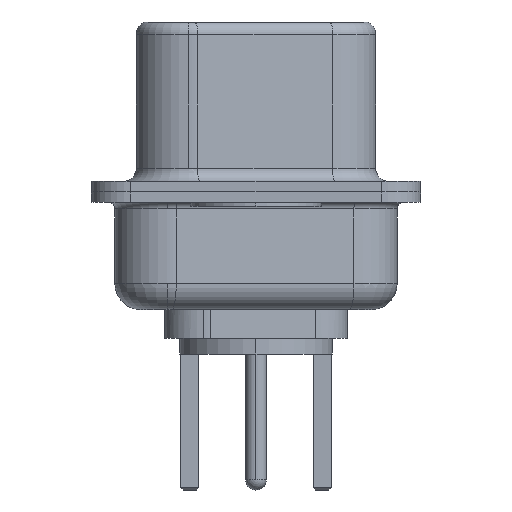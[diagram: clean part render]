
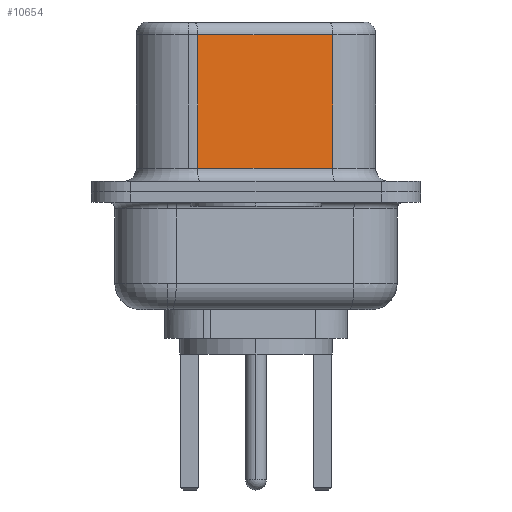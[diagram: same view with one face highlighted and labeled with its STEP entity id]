
A CAD part, left-side view. The second image highlights one B-rep face of the part: STEP entity #10654.
In plain terms, the highlighted planar face has unit normal (-0.985, -0.174, 0).
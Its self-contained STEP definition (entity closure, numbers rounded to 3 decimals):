
#803 = EDGE_LOOP ( 'NONE', ( #13712, #4889, #5428, #10880 ) ) ;
#1009 = VECTOR ( 'NONE', #5674, 1000. ) ;
#1105 = VECTOR ( 'NONE', #13350, 1000. ) ;
#1410 = VECTOR ( 'NONE', #2598, 1000. ) ;
#2425 = VERTEX_POINT ( 'NONE', #14596 ) ;
#2598 = DIRECTION ( 'NONE',  ( 0., 0., -1. ) ) ;
#3127 = CARTESIAN_POINT ( 'NONE',  ( 4.585, -2.927, 6.02 ) ) ;
#3784 = CARTESIAN_POINT ( 'NONE',  ( 3.675, 2.233, 6.52 ) ) ;
#3977 = CARTESIAN_POINT ( 'NONE',  ( 4.585, -2.927, 0.9 ) ) ;
#4550 = EDGE_CURVE ( 'NONE', #14071, #10435, #5283, .T. ) ;
#4889 = ORIENTED_EDGE ( 'NONE', *, *, #4550, .T. ) ;
#5022 = CARTESIAN_POINT ( 'NONE',  ( 4.585, -2.927, 6.02 ) ) ;
#5226 = LINE ( 'NONE', #3784, #1410 ) ;
#5283 = LINE ( 'NONE', #5022, #8017 ) ;
#5288 = EDGE_CURVE ( 'NONE', #14071, #11242, #10866, .T. ) ;
#5428 = ORIENTED_EDGE ( 'NONE', *, *, #9520, .T. ) ;
#5674 = DIRECTION ( 'NONE',  ( 0.174, -0.985, 0. ) ) ;
#5743 = DIRECTION ( 'NONE',  ( -0.174, 0.985, 0. ) ) ;
#5974 = EDGE_CURVE ( 'NONE', #2425, #11242, #7543, .T. ) ;
#6224 = AXIS2_PLACEMENT_3D ( 'NONE', #7383, #14578, #7479 ) ;
#6267 = PLANE ( 'NONE',  #6224 ) ;
#6866 = FACE_OUTER_BOUND ( 'NONE', #803, .T. ) ;
#7383 = CARTESIAN_POINT ( 'NONE',  ( 4.585, -2.927, 6.52 ) ) ;
#7479 = DIRECTION ( 'NONE',  ( -0.174, 0.985, 0. ) ) ;
#7543 = LINE ( 'NONE', #3977, #1009 ) ;
#8017 = VECTOR ( 'NONE', #5743, 1000. ) ;
#9520 = EDGE_CURVE ( 'NONE', #10435, #2425, #5226, .T. ) ;
#9566 = CARTESIAN_POINT ( 'NONE',  ( 3.675, 2.233, 6.02 ) ) ;
#10435 = VERTEX_POINT ( 'NONE', #9566 ) ;
#10654 = ADVANCED_FACE ( 'NONE', ( #6866 ), #6267, .F. ) ;
#10866 = LINE ( 'NONE', #13086, #1105 ) ;
#10880 = ORIENTED_EDGE ( 'NONE', *, *, #5974, .T. ) ;
#10966 = CARTESIAN_POINT ( 'NONE',  ( 4.585, -2.927, 0.9 ) ) ;
#11242 = VERTEX_POINT ( 'NONE', #10966 ) ;
#13086 = CARTESIAN_POINT ( 'NONE',  ( 4.585, -2.927, 6.52 ) ) ;
#13350 = DIRECTION ( 'NONE',  ( 0., 0., -1. ) ) ;
#13712 = ORIENTED_EDGE ( 'NONE', *, *, #5288, .F. ) ;
#14071 = VERTEX_POINT ( 'NONE', #3127 ) ;
#14578 = DIRECTION ( 'NONE',  ( 0.985, 0.174, 0. ) ) ;
#14596 = CARTESIAN_POINT ( 'NONE',  ( 3.675, 2.233, 0.9 ) ) ;
